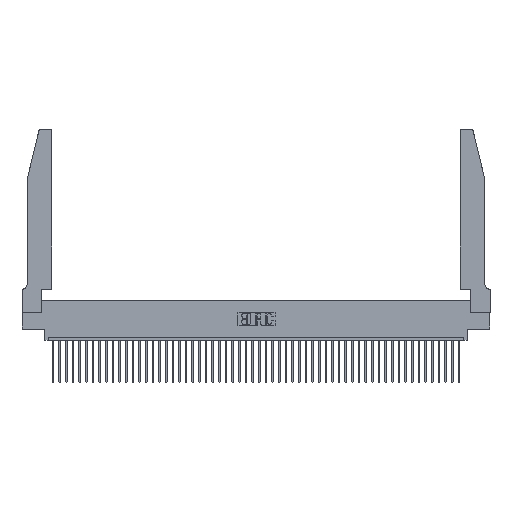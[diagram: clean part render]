
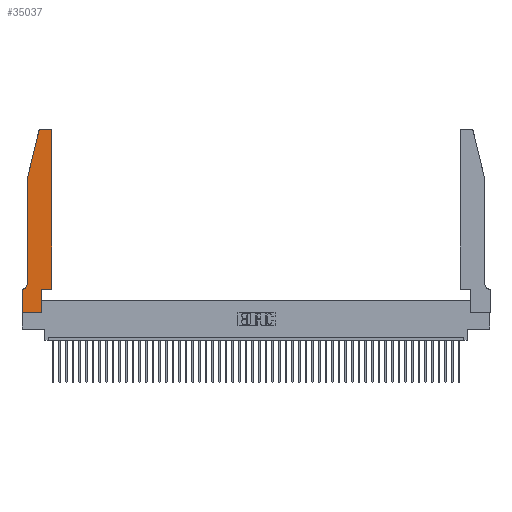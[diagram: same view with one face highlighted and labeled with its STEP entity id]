
A CAD part, top view. The second image highlights one B-rep face of the part: STEP entity #35037.
In plain terms, the highlighted planar face has unit normal (0, 0, 1).
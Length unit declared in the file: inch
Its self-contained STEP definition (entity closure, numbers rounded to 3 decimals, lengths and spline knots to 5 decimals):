
#170 = VECTOR ( 'NONE', #4684, 39.37008 ) ;
#610 = CARTESIAN_POINT ( 'NONE',  ( 0., 0., 0.37 ) ) ;
#1279 = EDGE_CURVE ( 'NONE', #6533, #10130, #3452, .T. ) ;
#1296 = LINE ( 'NONE', #38252, #170 ) ;
#1671 = DIRECTION ( 'NONE',  ( -1., 0., 0. ) ) ;
#2076 = ORIENTED_EDGE ( 'NONE', *, *, #35522, .T. ) ;
#3452 = LINE ( 'NONE', #27218, #14622 ) ;
#3729 = EDGE_CURVE ( 'NONE', #29560, #39896, #45627, .T. ) ;
#4572 = VERTEX_POINT ( 'NONE', #30662 ) ;
#4641 = CARTESIAN_POINT ( 'NONE',  ( 0.25487, 2.72718, 0.37 ) ) ;
#4684 = DIRECTION ( 'NONE',  ( 1., 0., 0. ) ) ;
#4844 = VECTOR ( 'NONE', #10612, 39.37008 ) ;
#5054 = DIRECTION ( 'NONE',  ( 0., 1., 0. ) ) ;
#5242 = CARTESIAN_POINT ( 'NONE',  ( 0., 0.35, 0.37 ) ) ;
#5511 = DIRECTION ( 'NONE',  ( 0., 0., 1. ) ) ;
#6298 = VERTEX_POINT ( 'NONE', #24747 ) ;
#6533 = VERTEX_POINT ( 'NONE', #34885 ) ;
#7731 = CIRCLE ( 'NONE', #28765, 0.07 ) ;
#8677 = VECTOR ( 'NONE', #26988, 39.37008 ) ;
#9603 = EDGE_CURVE ( 'NONE', #4572, #22439, #21953, .T. ) ;
#9667 = ORIENTED_EDGE ( 'NONE', *, *, #9603, .T. ) ;
#10130 = VERTEX_POINT ( 'NONE', #32959 ) ;
#10600 = VECTOR ( 'NONE', #15733, 39.37008 ) ;
#10612 = DIRECTION ( 'NONE',  ( 1., 0., 0. ) ) ;
#11461 = CARTESIAN_POINT ( 'NONE',  ( 0.0755, 2., 0.37 ) ) ;
#11475 = DIRECTION ( 'NONE',  ( 0., -1., 0. ) ) ;
#11734 = DIRECTION ( 'NONE',  ( 1., 0., 0. ) ) ;
#11785 = VECTOR ( 'NONE', #23104, 39.37008 ) ;
#12900 = VERTEX_POINT ( 'NONE', #21185 ) ;
#13025 = VECTOR ( 'NONE', #11475, 39.37008 ) ;
#13030 = VECTOR ( 'NONE', #30334, 39.37008 ) ;
#14622 = VECTOR ( 'NONE', #19953, 39.37008 ) ;
#14910 = AXIS2_PLACEMENT_3D ( 'NONE', #15392, #34700, #11734 ) ;
#15212 = VERTEX_POINT ( 'NONE', #41045 ) ;
#15392 = CARTESIAN_POINT ( 'NONE',  ( 0.284, 2.72, 0.37 ) ) ;
#15733 = DIRECTION ( 'NONE',  ( 0., -1., 0. ) ) ;
#16202 = ORIENTED_EDGE ( 'NONE', *, *, #17040, .T. ) ;
#16440 = CARTESIAN_POINT ( 'NONE',  ( 0., 0.35, 0.37 ) ) ;
#17040 = EDGE_CURVE ( 'NONE', #39896, #45636, #1296, .T. ) ;
#17617 = DIRECTION ( 'NONE',  ( 1., 0., 0. ) ) ;
#18283 = LINE ( 'NONE', #31451, #10600 ) ;
#18392 = CARTESIAN_POINT ( 'NONE',  ( 0.4505, 0.35, 0.37 ) ) ;
#18856 = ORIENTED_EDGE ( 'NONE', *, *, #28037, .T. ) ;
#19953 = DIRECTION ( 'NONE',  ( -1., 0., 0. ) ) ;
#19975 = VERTEX_POINT ( 'NONE', #48085 ) ;
#21185 = CARTESIAN_POINT ( 'NONE',  ( 0.0755, 2., 0.37 ) ) ;
#21558 = FACE_OUTER_BOUND ( 'NONE', #38323, .T. ) ;
#21953 = LINE ( 'NONE', #33080, #4844 ) ;
#22439 = VERTEX_POINT ( 'NONE', #18392 ) ;
#23025 = LINE ( 'NONE', #45676, #11785 ) ;
#23104 = DIRECTION ( 'NONE',  ( 0., 1., 0. ) ) ;
#23949 = ORIENTED_EDGE ( 'NONE', *, *, #48536, .T. ) ;
#24347 = PLANE ( 'NONE',  #39945 ) ;
#24377 = DIRECTION ( 'NONE',  ( 0., 0., -1. ) ) ;
#24747 = CARTESIAN_POINT ( 'NONE',  ( 0.0755, 0.42, 0.37 ) ) ;
#24860 = DIRECTION ( 'NONE',  ( 0., 0., 1. ) ) ;
#26988 = DIRECTION ( 'NONE',  ( -1., 0., 0. ) ) ;
#27218 = CARTESIAN_POINT ( 'NONE',  ( 0.2605, 2.75, 0.37 ) ) ;
#27333 = CIRCLE ( 'NONE', #14910, 0.03 ) ;
#27464 = ORIENTED_EDGE ( 'NONE', *, *, #1279, .T. ) ;
#28037 = EDGE_CURVE ( 'NONE', #12900, #6298, #18283, .T. ) ;
#28765 = AXIS2_PLACEMENT_3D ( 'NONE', #35312, #24377, #1671 ) ;
#29560 = VERTEX_POINT ( 'NONE', #5242 ) ;
#29639 = LINE ( 'NONE', #11461, #13030 ) ;
#30064 = ORIENTED_EDGE ( 'NONE', *, *, #35174, .T. ) ;
#30334 = DIRECTION ( 'NONE',  ( -0.239, -0.971, 0. ) ) ;
#30662 = CARTESIAN_POINT ( 'NONE',  ( 0.2865, 0.35, 0.37 ) ) ;
#30962 = CARTESIAN_POINT ( 'NONE',  ( 0.0755, 0.35, 0.37 ) ) ;
#31451 = CARTESIAN_POINT ( 'NONE',  ( 0.0755, 2., 0.37 ) ) ;
#32959 = CARTESIAN_POINT ( 'NONE',  ( 0.284, 2.75, 0.37 ) ) ;
#33080 = CARTESIAN_POINT ( 'NONE',  ( 0.4505, 0.35, 0.37 ) ) ;
#33320 = ORIENTED_EDGE ( 'NONE', *, *, #35663, .T. ) ;
#33679 = CARTESIAN_POINT ( 'NONE',  ( 0.2865, 0., 0.37 ) ) ;
#34246 = ORIENTED_EDGE ( 'NONE', *, *, #43443, .T. ) ;
#34667 = ORIENTED_EDGE ( 'NONE', *, *, #39967, .T. ) ;
#34700 = DIRECTION ( 'NONE',  ( 0., 0., 1. ) ) ;
#34885 = CARTESIAN_POINT ( 'NONE',  ( 0.4205, 2.75, 0.37 ) ) ;
#35037 = ADVANCED_FACE ( 'NONE', ( #21558 ), #24347, .T. ) ;
#35174 = EDGE_CURVE ( 'NONE', #19975, #6533, #41685, .T. ) ;
#35312 = CARTESIAN_POINT ( 'NONE',  ( 0.0055, 0.42, 0.37 ) ) ;
#35522 = EDGE_CURVE ( 'NONE', #22439, #19975, #38675, .T. ) ;
#35663 = EDGE_CURVE ( 'NONE', #10130, #46388, #27333, .T. ) ;
#36609 = ORIENTED_EDGE ( 'NONE', *, *, #3729, .T. ) ;
#38079 = VECTOR ( 'NONE', #5054, 39.37008 ) ;
#38252 = CARTESIAN_POINT ( 'NONE',  ( 0., 0., 0.37 ) ) ;
#38323 = EDGE_LOOP ( 'NONE', ( #27464, #33320, #42295, #18856, #23949, #34667, #36609, #16202, #34246, #9667, #2076, #30064 ) ) ;
#38675 = LINE ( 'NONE', #46048, #38079 ) ;
#39896 = VERTEX_POINT ( 'NONE', #42410 ) ;
#39945 = AXIS2_PLACEMENT_3D ( 'NONE', #16440, #24860, #17617 ) ;
#39967 = EDGE_CURVE ( 'NONE', #15212, #29560, #43621, .T. ) ;
#41045 = CARTESIAN_POINT ( 'NONE',  ( 0.0055, 0.35, 0.37 ) ) ;
#41685 = CIRCLE ( 'NONE', #45363, 0.03 ) ;
#42295 = ORIENTED_EDGE ( 'NONE', *, *, #48859, .T. ) ;
#42410 = CARTESIAN_POINT ( 'NONE',  ( 0., 0., 0.37 ) ) ;
#43443 = EDGE_CURVE ( 'NONE', #45636, #4572, #23025, .T. ) ;
#43551 = CARTESIAN_POINT ( 'NONE',  ( 0.4205, 2.72, 0.37 ) ) ;
#43621 = LINE ( 'NONE', #30962, #8677 ) ;
#45363 = AXIS2_PLACEMENT_3D ( 'NONE', #43551, #5511, #47343 ) ;
#45627 = LINE ( 'NONE', #610, #13025 ) ;
#45636 = VERTEX_POINT ( 'NONE', #33679 ) ;
#45676 = CARTESIAN_POINT ( 'NONE',  ( 0.2865, 0.35, 0.37 ) ) ;
#46048 = CARTESIAN_POINT ( 'NONE',  ( 0.4505, 0.35, 0.37 ) ) ;
#46388 = VERTEX_POINT ( 'NONE', #4641 ) ;
#47343 = DIRECTION ( 'NONE',  ( 1., 0., 0. ) ) ;
#48085 = CARTESIAN_POINT ( 'NONE',  ( 0.4505, 2.72, 0.37 ) ) ;
#48536 = EDGE_CURVE ( 'NONE', #6298, #15212, #7731, .T. ) ;
#48859 = EDGE_CURVE ( 'NONE', #46388, #12900, #29639, .T. ) ;
